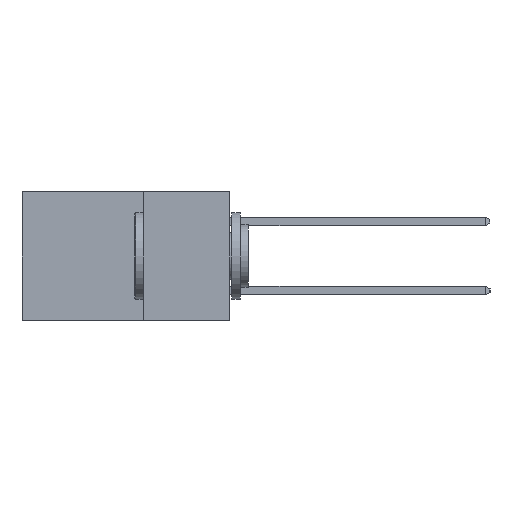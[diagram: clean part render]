
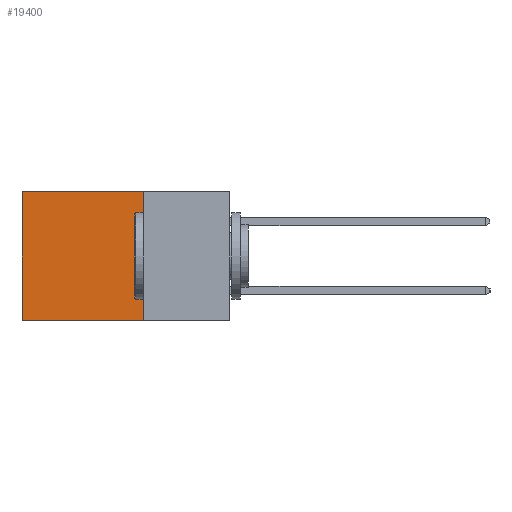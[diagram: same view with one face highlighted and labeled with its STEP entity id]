
A CAD part, left-side view. The second image highlights one B-rep face of the part: STEP entity #19400.
In plain terms, the highlighted planar face has unit normal (-1, 0, 0).
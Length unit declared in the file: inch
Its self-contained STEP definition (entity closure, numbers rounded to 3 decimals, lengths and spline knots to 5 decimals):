
#821 = LINE ( 'NONE', #4416, #20174 ) ;
#1778 = CARTESIAN_POINT ( 'NONE',  ( 0.2615, 0.6, -0.37 ) ) ;
#3147 = DIRECTION ( 'NONE',  ( 1., 0., 0. ) ) ;
#3427 = VERTEX_POINT ( 'NONE', #7977 ) ;
#3941 = VERTEX_POINT ( 'NONE', #1778 ) ;
#4054 = VECTOR ( 'NONE', #17053, 39.37008 ) ;
#4416 = CARTESIAN_POINT ( 'NONE',  ( 0.2615, 0.6, -0.37 ) ) ;
#4521 = VECTOR ( 'NONE', #5006, 39.37008 ) ;
#4571 = CARTESIAN_POINT ( 'NONE',  ( 0.2615, 0.25, 0. ) ) ;
#4770 = CARTESIAN_POINT ( 'NONE',  ( 0.2615, 0.25, -0.37 ) ) ;
#5006 = DIRECTION ( 'NONE',  ( 0., 0., -1. ) ) ;
#5603 = CARTESIAN_POINT ( 'NONE',  ( 0.2615, 0.25, -0.37 ) ) ;
#7019 = CARTESIAN_POINT ( 'NONE',  ( 0.2615, 0.6, 0. ) ) ;
#7543 = VERTEX_POINT ( 'NONE', #5603 ) ;
#7555 = DIRECTION ( 'NONE',  ( 0., 0., -1. ) ) ;
#7977 = CARTESIAN_POINT ( 'NONE',  ( 0.2615, 0.25, 0. ) ) ;
#8708 = FACE_OUTER_BOUND ( 'NONE', #17175, .T. ) ;
#9179 = ORIENTED_EDGE ( 'NONE', *, *, #18564, .T. ) ;
#9236 = ORIENTED_EDGE ( 'NONE', *, *, #9655, .T. ) ;
#9359 = PLANE ( 'NONE',  #11260 ) ;
#9655 = EDGE_CURVE ( 'NONE', #3427, #14784, #12343, .T. ) ;
#11260 = AXIS2_PLACEMENT_3D ( 'NONE', #12483, #3147, #14070 ) ;
#11610 = EDGE_CURVE ( 'NONE', #7543, #3941, #17918, .T. ) ;
#12343 = LINE ( 'NONE', #4571, #4054 ) ;
#12483 = CARTESIAN_POINT ( 'NONE',  ( 0.2615, 0.25, -0.37 ) ) ;
#13259 = VECTOR ( 'NONE', #13867, 39.37008 ) ;
#13867 = DIRECTION ( 'NONE',  ( 0., 1., 0. ) ) ;
#14070 = DIRECTION ( 'NONE',  ( 0., 0., -1. ) ) ;
#14411 = ORIENTED_EDGE ( 'NONE', *, *, #19877, .F. ) ;
#14784 = VERTEX_POINT ( 'NONE', #7019 ) ;
#16955 = LINE ( 'NONE', #4770, #4521 ) ;
#17003 = CARTESIAN_POINT ( 'NONE',  ( 0.2615, 0.25, -0.37 ) ) ;
#17053 = DIRECTION ( 'NONE',  ( 0., 1., 0. ) ) ;
#17175 = EDGE_LOOP ( 'NONE', ( #9179, #19576, #14411, #9236 ) ) ;
#17918 = LINE ( 'NONE', #17003, #13259 ) ;
#18564 = EDGE_CURVE ( 'NONE', #14784, #3941, #821, .T. ) ;
#19400 = ADVANCED_FACE ( 'NONE', ( #8708 ), #9359, .F. ) ;
#19576 = ORIENTED_EDGE ( 'NONE', *, *, #11610, .F. ) ;
#19877 = EDGE_CURVE ( 'NONE', #3427, #7543, #16955, .T. ) ;
#20174 = VECTOR ( 'NONE', #7555, 39.37008 ) ;
